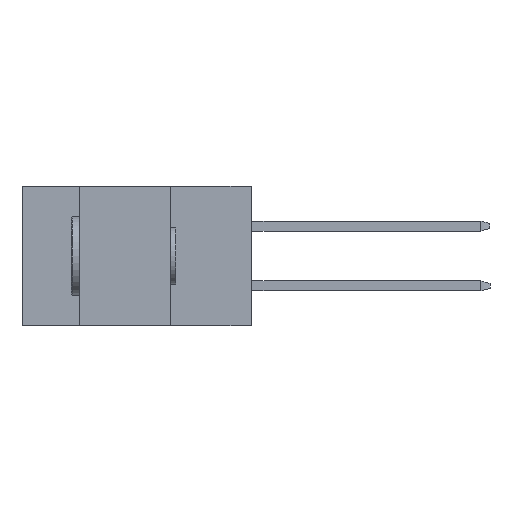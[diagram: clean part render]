
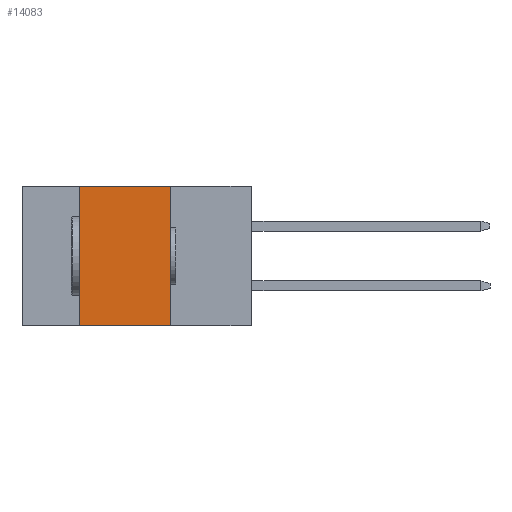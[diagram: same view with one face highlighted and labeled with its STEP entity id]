
A CAD part, left-side view. The second image highlights one B-rep face of the part: STEP entity #14083.
In plain terms, the highlighted planar face has unit normal (-1, 0, 0).
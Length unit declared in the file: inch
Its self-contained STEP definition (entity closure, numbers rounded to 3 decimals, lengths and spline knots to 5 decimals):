
#339 = CARTESIAN_POINT ( 'NONE',  ( 0., 0.54, -0.437 ) ) ;
#623 = DIRECTION ( 'NONE',  ( 0., -1., 0. ) ) ;
#858 = ORIENTED_EDGE ( 'NONE', *, *, #9709, .F. ) ;
#860 = EDGE_CURVE ( 'NONE', #10004, #9407, #5712, .T. ) ;
#952 = VERTEX_POINT ( 'NONE', #15774 ) ;
#1537 = LINE ( 'NONE', #14717, #13374 ) ;
#2475 = FACE_OUTER_BOUND ( 'NONE', #6462, .T. ) ;
#3269 = AXIS2_PLACEMENT_3D ( 'NONE', #11370, #8409, #3994 ) ;
#3994 = DIRECTION ( 'NONE',  ( 0., 0., -1. ) ) ;
#4524 = VECTOR ( 'NONE', #8512, 39.37008 ) ;
#4882 = CARTESIAN_POINT ( 'NONE',  ( 0., 0.72, -0.437 ) ) ;
#5712 = LINE ( 'NONE', #11480, #4524 ) ;
#5881 = CARTESIAN_POINT ( 'NONE',  ( 0., 0.254, -0.437 ) ) ;
#6172 = EDGE_CURVE ( 'NONE', #7525, #10004, #1537, .T. ) ;
#6462 = EDGE_LOOP ( 'NONE', ( #858, #17497, #13935, #16720 ) ) ;
#7038 = LINE ( 'NONE', #5881, #18144 ) ;
#7354 = DIRECTION ( 'NONE',  ( 0., 0., 1. ) ) ;
#7525 = VERTEX_POINT ( 'NONE', #339 ) ;
#8409 = DIRECTION ( 'NONE',  ( 1., 0., 0. ) ) ;
#8508 = PLANE ( 'NONE',  #3269 ) ;
#8512 = DIRECTION ( 'NONE',  ( 0., -1., 0. ) ) ;
#9407 = VERTEX_POINT ( 'NONE', #17483 ) ;
#9709 = EDGE_CURVE ( 'NONE', #9407, #952, #7038, .T. ) ;
#10004 = VERTEX_POINT ( 'NONE', #18595 ) ;
#11370 = CARTESIAN_POINT ( 'NONE',  ( 0., 0.72, 0. ) ) ;
#11480 = CARTESIAN_POINT ( 'NONE',  ( 0., 0.72, 0. ) ) ;
#13374 = VECTOR ( 'NONE', #7354, 39.37008 ) ;
#13935 = ORIENTED_EDGE ( 'NONE', *, *, #6172, .F. ) ;
#14083 = ADVANCED_FACE ( 'NONE', ( #2475 ), #8508, .F. ) ;
#14406 = DIRECTION ( 'NONE',  ( 0., 0., -1. ) ) ;
#14717 = CARTESIAN_POINT ( 'NONE',  ( 0., 0.54, -0.437 ) ) ;
#14853 = EDGE_CURVE ( 'NONE', #7525, #952, #18290, .T. ) ;
#15774 = CARTESIAN_POINT ( 'NONE',  ( 0., 0.254, -0.437 ) ) ;
#16720 = ORIENTED_EDGE ( 'NONE', *, *, #14853, .T. ) ;
#17483 = CARTESIAN_POINT ( 'NONE',  ( 0., 0.254, 0. ) ) ;
#17497 = ORIENTED_EDGE ( 'NONE', *, *, #860, .F. ) ;
#18144 = VECTOR ( 'NONE', #14406, 39.37008 ) ;
#18290 = LINE ( 'NONE', #4882, #18411 ) ;
#18411 = VECTOR ( 'NONE', #623, 39.37008 ) ;
#18595 = CARTESIAN_POINT ( 'NONE',  ( 0., 0.54, 0. ) ) ;
